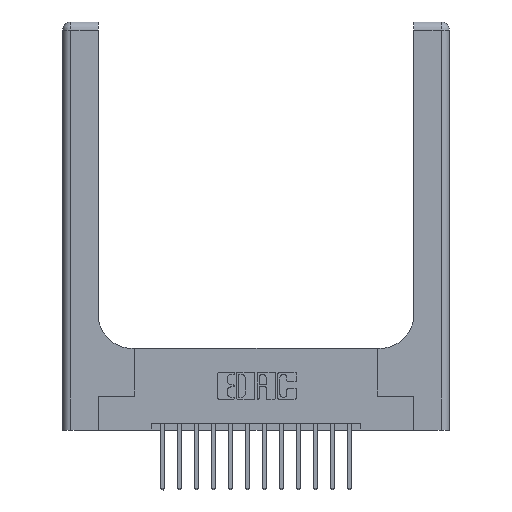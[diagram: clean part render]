
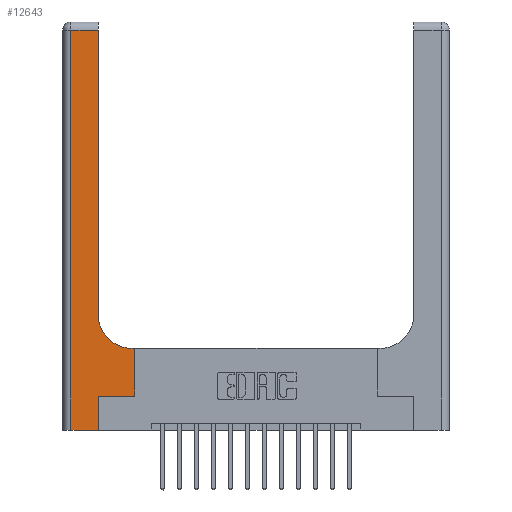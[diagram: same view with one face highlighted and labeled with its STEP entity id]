
A CAD part, top view. The second image highlights one B-rep face of the part: STEP entity #12643.
In plain terms, the highlighted planar face has unit normal (0, 0, 1).
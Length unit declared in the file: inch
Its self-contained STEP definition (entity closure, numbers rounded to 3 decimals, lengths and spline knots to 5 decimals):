
#94 = LINE ( 'NONE', #3336, #12659 ) ;
#480 = PLANE ( 'NONE',  #6200 ) ;
#691 = VERTEX_POINT ( 'NONE', #7555 ) ;
#719 = EDGE_CURVE ( 'NONE', #8819, #11408, #15012, .T. ) ;
#838 = CARTESIAN_POINT ( 'NONE',  ( 0., 2.94, 0.37 ) ) ;
#942 = EDGE_CURVE ( 'NONE', #9781, #1098, #12719, .T. ) ;
#1098 = VERTEX_POINT ( 'NONE', #8724 ) ;
#1599 = CARTESIAN_POINT ( 'NONE',  ( 0.26, 2.94, 0.37 ) ) ;
#1616 = ORIENTED_EDGE ( 'NONE', *, *, #3369, .T. ) ;
#2129 = VERTEX_POINT ( 'NONE', #7739 ) ;
#2175 = DIRECTION ( 'NONE',  ( 0., 1., 0. ) ) ;
#2568 = CARTESIAN_POINT ( 'NONE',  ( 0.51, 0.85, 0.37 ) ) ;
#2617 = AXIS2_PLACEMENT_3D ( 'NONE', #2568, #6297, #15468 ) ;
#2631 = CARTESIAN_POINT ( 'NONE',  ( 0.528, 0.25, 0.37 ) ) ;
#3336 = CARTESIAN_POINT ( 'NONE',  ( 0.06, 3., 0.37 ) ) ;
#3369 = EDGE_CURVE ( 'NONE', #14008, #8819, #94, .T. ) ;
#3545 = CARTESIAN_POINT ( 'NONE',  ( 0.06, 2.94, 0.37 ) ) ;
#3631 = ORIENTED_EDGE ( 'NONE', *, *, #719, .T. ) ;
#3975 = DIRECTION ( 'NONE',  ( 0., 1., 0. ) ) ;
#4104 = DIRECTION ( 'NONE',  ( -1., 0., 0. ) ) ;
#4212 = CARTESIAN_POINT ( 'NONE',  ( 0.265, 0., 0.37 ) ) ;
#4605 = CIRCLE ( 'NONE', #2617, 0.25 ) ;
#5145 = VECTOR ( 'NONE', #4104, 39.37008 ) ;
#5344 = CARTESIAN_POINT ( 'NONE',  ( 0.26, 0.85, 0.37 ) ) ;
#5393 = CARTESIAN_POINT ( 'NONE',  ( 0.265, 0.25, 0.37 ) ) ;
#5497 = EDGE_CURVE ( 'NONE', #8522, #14008, #15687, .T. ) ;
#5597 = DIRECTION ( 'NONE',  ( 0., -1., 0. ) ) ;
#5905 = ORIENTED_EDGE ( 'NONE', *, *, #15763, .T. ) ;
#5966 = LINE ( 'NONE', #9822, #9275 ) ;
#5978 = FACE_OUTER_BOUND ( 'NONE', #12213, .T. ) ;
#6020 = EDGE_CURVE ( 'NONE', #11408, #9781, #5966, .T. ) ;
#6200 = AXIS2_PLACEMENT_3D ( 'NONE', #10938, #16157, #9610 ) ;
#6224 = CARTESIAN_POINT ( 'NONE',  ( 0.265, 0.25, 0.37 ) ) ;
#6297 = DIRECTION ( 'NONE',  ( 0., 0., -1. ) ) ;
#6935 = VECTOR ( 'NONE', #11837, 39.37008 ) ;
#7229 = EDGE_CURVE ( 'NONE', #15836, #8522, #15213, .T. ) ;
#7287 = EDGE_CURVE ( 'NONE', #691, #2129, #13800, .T. ) ;
#7555 = CARTESIAN_POINT ( 'NONE',  ( 0.528, 0.6, 0.37 ) ) ;
#7739 = CARTESIAN_POINT ( 'NONE',  ( 0.51, 0.6, 0.37 ) ) ;
#7802 = VECTOR ( 'NONE', #11646, 39.37008 ) ;
#8167 = CARTESIAN_POINT ( 'NONE',  ( 0., 0., 0.37 ) ) ;
#8245 = VECTOR ( 'NONE', #8891, 39.37008 ) ;
#8427 = ORIENTED_EDGE ( 'NONE', *, *, #7287, .T. ) ;
#8454 = EDGE_CURVE ( 'NONE', #1098, #691, #15638, .T. ) ;
#8522 = VERTEX_POINT ( 'NONE', #1599 ) ;
#8724 = CARTESIAN_POINT ( 'NONE',  ( 0.528, 0.25, 0.37 ) ) ;
#8819 = VERTEX_POINT ( 'NONE', #8861 ) ;
#8861 = CARTESIAN_POINT ( 'NONE',  ( 0.06, 0., 0.37 ) ) ;
#8891 = DIRECTION ( 'NONE',  ( -1., 0., 0. ) ) ;
#9275 = VECTOR ( 'NONE', #2175, 39.37008 ) ;
#9542 = ORIENTED_EDGE ( 'NONE', *, *, #942, .T. ) ;
#9610 = DIRECTION ( 'NONE',  ( -1., 0., 0. ) ) ;
#9781 = VERTEX_POINT ( 'NONE', #6224 ) ;
#9822 = CARTESIAN_POINT ( 'NONE',  ( 0.265, 0., 0.37 ) ) ;
#10938 = CARTESIAN_POINT ( 'NONE',  ( 0., 3., 0.37 ) ) ;
#11145 = ORIENTED_EDGE ( 'NONE', *, *, #8454, .T. ) ;
#11289 = VECTOR ( 'NONE', #3975, 39.37008 ) ;
#11408 = VERTEX_POINT ( 'NONE', #4212 ) ;
#11646 = DIRECTION ( 'NONE',  ( 0., 1., 0. ) ) ;
#11794 = ORIENTED_EDGE ( 'NONE', *, *, #5497, .T. ) ;
#11837 = DIRECTION ( 'NONE',  ( 1., 0., 0. ) ) ;
#12213 = EDGE_LOOP ( 'NONE', ( #15864, #11794, #1616, #3631, #14489, #9542, #11145, #8427, #5905 ) ) ;
#12643 = ADVANCED_FACE ( 'NONE', ( #5978 ), #480, .F. ) ;
#12659 = VECTOR ( 'NONE', #5597, 39.37008 ) ;
#12719 = LINE ( 'NONE', #5393, #6935 ) ;
#12919 = CARTESIAN_POINT ( 'NONE',  ( 0.26, 3., 0.37 ) ) ;
#13800 = LINE ( 'NONE', #16032, #5145 ) ;
#14008 = VERTEX_POINT ( 'NONE', #3545 ) ;
#14489 = ORIENTED_EDGE ( 'NONE', *, *, #6020, .T. ) ;
#15012 = LINE ( 'NONE', #8167, #15837 ) ;
#15213 = LINE ( 'NONE', #12919, #7802 ) ;
#15468 = DIRECTION ( 'NONE',  ( 1., 0., 0. ) ) ;
#15638 = LINE ( 'NONE', #2631, #11289 ) ;
#15687 = LINE ( 'NONE', #838, #8245 ) ;
#15763 = EDGE_CURVE ( 'NONE', #2129, #15836, #4605, .T. ) ;
#15836 = VERTEX_POINT ( 'NONE', #5344 ) ;
#15837 = VECTOR ( 'NONE', #15919, 39.37008 ) ;
#15864 = ORIENTED_EDGE ( 'NONE', *, *, #7229, .T. ) ;
#15919 = DIRECTION ( 'NONE',  ( 1., 0., 0. ) ) ;
#16032 = CARTESIAN_POINT ( 'NONE',  ( 0.26, 0.6, 0.37 ) ) ;
#16157 = DIRECTION ( 'NONE',  ( 0., 0., -1. ) ) ;
